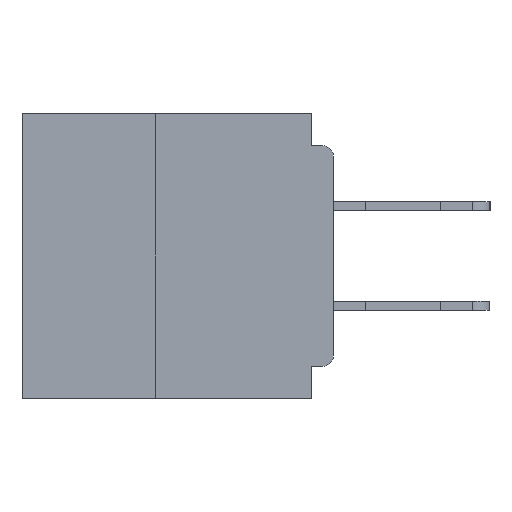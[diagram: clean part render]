
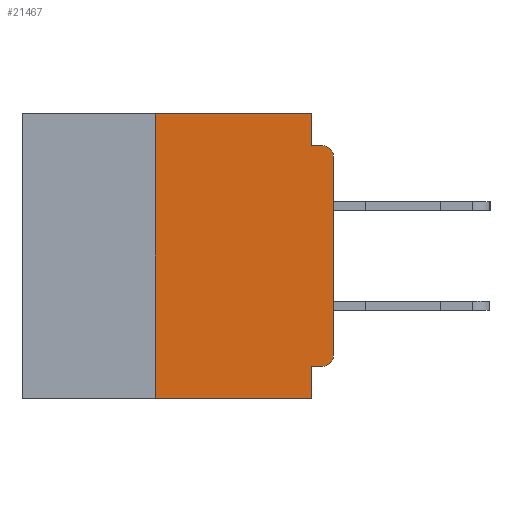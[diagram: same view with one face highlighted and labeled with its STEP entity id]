
A CAD part, left-side view. The second image highlights one B-rep face of the part: STEP entity #21467.
In plain terms, the highlighted planar face has unit normal (-1, 0, 0).
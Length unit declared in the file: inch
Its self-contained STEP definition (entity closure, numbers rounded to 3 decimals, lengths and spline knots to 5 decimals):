
#212 = ORIENTED_EDGE ( 'NONE', *, *, #21459, .F. ) ;
#314 = CARTESIAN_POINT ( 'NONE',  ( 0., 0.031, 0. ) ) ;
#1347 = EDGE_LOOP ( 'NONE', ( #4429, #32318, #212, #3685, #7725, #4936, #39510, #24696, #27325, #12631 ) ) ;
#1781 = CARTESIAN_POINT ( 'NONE',  ( 0., 0., -0.06 ) ) ;
#1865 = DIRECTION ( 'NONE',  ( 0., 0., -1. ) ) ;
#3379 = CIRCLE ( 'NONE', #32879, 0.015 ) ;
#3685 = ORIENTED_EDGE ( 'NONE', *, *, #43023, .F. ) ;
#4008 = LINE ( 'NONE', #25801, #36933 ) ;
#4429 = ORIENTED_EDGE ( 'NONE', *, *, #30824, .T. ) ;
#4936 = ORIENTED_EDGE ( 'NONE', *, *, #37138, .F. ) ;
#5712 = CARTESIAN_POINT ( 'NONE',  ( 0., 0.031, -0.4 ) ) ;
#6033 = DIRECTION ( 'NONE',  ( 0., -1., 0. ) ) ;
#7304 = VECTOR ( 'NONE', #17323, 39.37008 ) ;
#7725 = ORIENTED_EDGE ( 'NONE', *, *, #27133, .F. ) ;
#7884 = CARTESIAN_POINT ( 'NONE',  ( 0., 0.015, -0.06 ) ) ;
#11268 = VECTOR ( 'NONE', #43178, 39.37008 ) ;
#12236 = DIRECTION ( 'NONE',  ( 0., 0., -1. ) ) ;
#12631 = ORIENTED_EDGE ( 'NONE', *, *, #43439, .T. ) ;
#14232 = VERTEX_POINT ( 'NONE', #26985 ) ;
#14714 = AXIS2_PLACEMENT_3D ( 'NONE', #23380, #27658, #1865 ) ;
#15633 = VERTEX_POINT ( 'NONE', #1781 ) ;
#15743 = FACE_OUTER_BOUND ( 'NONE', #1347, .T. ) ;
#16026 = DIRECTION ( 'NONE',  ( -1., 0., 0. ) ) ;
#16431 = DIRECTION ( 'NONE',  ( 0., 0., 1. ) ) ;
#17108 = VECTOR ( 'NONE', #6033, 39.37008 ) ;
#17323 = DIRECTION ( 'NONE',  ( 0., 0., -1. ) ) ;
#17520 = VECTOR ( 'NONE', #55054, 39.37008 ) ;
#17716 = AXIS2_PLACEMENT_3D ( 'NONE', #7884, #37885, #12236 ) ;
#18793 = LINE ( 'NONE', #38621, #7304 ) ;
#19393 = EDGE_CURVE ( 'NONE', #14232, #39694, #25411, .T. ) ;
#19512 = VECTOR ( 'NONE', #51767, 39.37008 ) ;
#21459 = EDGE_CURVE ( 'NONE', #41559, #49579, #27140, .T. ) ;
#21467 = ADVANCED_FACE ( 'NONE', ( #15743 ), #48964, .F. ) ;
#23380 = CARTESIAN_POINT ( 'NONE',  ( 0., 0.437, 0. ) ) ;
#23886 = EDGE_CURVE ( 'NONE', #15633, #49579, #38312, .T. ) ;
#24687 = CARTESIAN_POINT ( 'NONE',  ( 0., 0.015, -0.355 ) ) ;
#24696 = ORIENTED_EDGE ( 'NONE', *, *, #37814, .F. ) ;
#25228 = CARTESIAN_POINT ( 'NONE',  ( 0., 0., -0.355 ) ) ;
#25411 = LINE ( 'NONE', #38876, #11268 ) ;
#25801 = CARTESIAN_POINT ( 'NONE',  ( 0., 0.437, 0. ) ) ;
#26691 = VERTEX_POINT ( 'NONE', #35693 ) ;
#26985 = CARTESIAN_POINT ( 'NONE',  ( 0., 0.25, -0.4 ) ) ;
#27133 = EDGE_CURVE ( 'NONE', #51866, #55450, #4008, .T. ) ;
#27140 = LINE ( 'NONE', #31758, #17108 ) ;
#27325 = ORIENTED_EDGE ( 'NONE', *, *, #50868, .F. ) ;
#27658 = DIRECTION ( 'NONE',  ( 1., 0., 0. ) ) ;
#28902 = LINE ( 'NONE', #25228, #17520 ) ;
#29171 = CARTESIAN_POINT ( 'NONE',  ( 0., 0.25, -0.4 ) ) ;
#29571 = VECTOR ( 'NONE', #16431, 39.37008 ) ;
#30824 = EDGE_CURVE ( 'NONE', #26691, #15633, #43292, .T. ) ;
#31758 = CARTESIAN_POINT ( 'NONE',  ( 0., 0., -0.045 ) ) ;
#32318 = ORIENTED_EDGE ( 'NONE', *, *, #23886, .T. ) ;
#32879 = AXIS2_PLACEMENT_3D ( 'NONE', #41672, #16026, #45984 ) ;
#34399 = VERTEX_POINT ( 'NONE', #24687 ) ;
#35693 = CARTESIAN_POINT ( 'NONE',  ( 0., 0., -0.34 ) ) ;
#36933 = VECTOR ( 'NONE', #42599, 39.37008 ) ;
#37138 = EDGE_CURVE ( 'NONE', #14232, #51866, #52257, .T. ) ;
#37814 = EDGE_CURVE ( 'NONE', #50348, #39694, #18793, .T. ) ;
#37885 = DIRECTION ( 'NONE',  ( -1., 0., 0. ) ) ;
#37948 = CARTESIAN_POINT ( 'NONE',  ( 0., 0.25, 0. ) ) ;
#38312 = CIRCLE ( 'NONE', #17716, 0.015 ) ;
#38621 = CARTESIAN_POINT ( 'NONE',  ( 0., 0.031, -0.4 ) ) ;
#38701 = CARTESIAN_POINT ( 'NONE',  ( 0., 0.031, -0.355 ) ) ;
#38876 = CARTESIAN_POINT ( 'NONE',  ( 0., 0.437, -0.4 ) ) ;
#39265 = VECTOR ( 'NONE', #41709, 39.37008 ) ;
#39510 = ORIENTED_EDGE ( 'NONE', *, *, #19393, .T. ) ;
#39694 = VERTEX_POINT ( 'NONE', #5712 ) ;
#41559 = VERTEX_POINT ( 'NONE', #44717 ) ;
#41672 = CARTESIAN_POINT ( 'NONE',  ( 0., 0.015, -0.34 ) ) ;
#41709 = DIRECTION ( 'NONE',  ( 0., 0., 1. ) ) ;
#42599 = DIRECTION ( 'NONE',  ( 0., -1., 0. ) ) ;
#43023 = EDGE_CURVE ( 'NONE', #55450, #41559, #53540, .T. ) ;
#43178 = DIRECTION ( 'NONE',  ( 0., -1., 0. ) ) ;
#43292 = LINE ( 'NONE', #46023, #39265 ) ;
#43439 = EDGE_CURVE ( 'NONE', #34399, #26691, #3379, .T. ) ;
#44717 = CARTESIAN_POINT ( 'NONE',  ( 0., 0.031, -0.045 ) ) ;
#45984 = DIRECTION ( 'NONE',  ( 0., 0., -1. ) ) ;
#46023 = CARTESIAN_POINT ( 'NONE',  ( 0., 0., 0. ) ) ;
#47499 = CARTESIAN_POINT ( 'NONE',  ( 0., 0.031, 0. ) ) ;
#48964 = PLANE ( 'NONE',  #14714 ) ;
#49579 = VERTEX_POINT ( 'NONE', #50742 ) ;
#50348 = VERTEX_POINT ( 'NONE', #38701 ) ;
#50742 = CARTESIAN_POINT ( 'NONE',  ( 0., 0.015, -0.045 ) ) ;
#50868 = EDGE_CURVE ( 'NONE', #34399, #50348, #28902, .T. ) ;
#51767 = DIRECTION ( 'NONE',  ( 0., 0., -1. ) ) ;
#51866 = VERTEX_POINT ( 'NONE', #37948 ) ;
#52257 = LINE ( 'NONE', #29171, #29571 ) ;
#53540 = LINE ( 'NONE', #47499, #19512 ) ;
#55054 = DIRECTION ( 'NONE',  ( 0., 1., 0. ) ) ;
#55450 = VERTEX_POINT ( 'NONE', #314 ) ;
